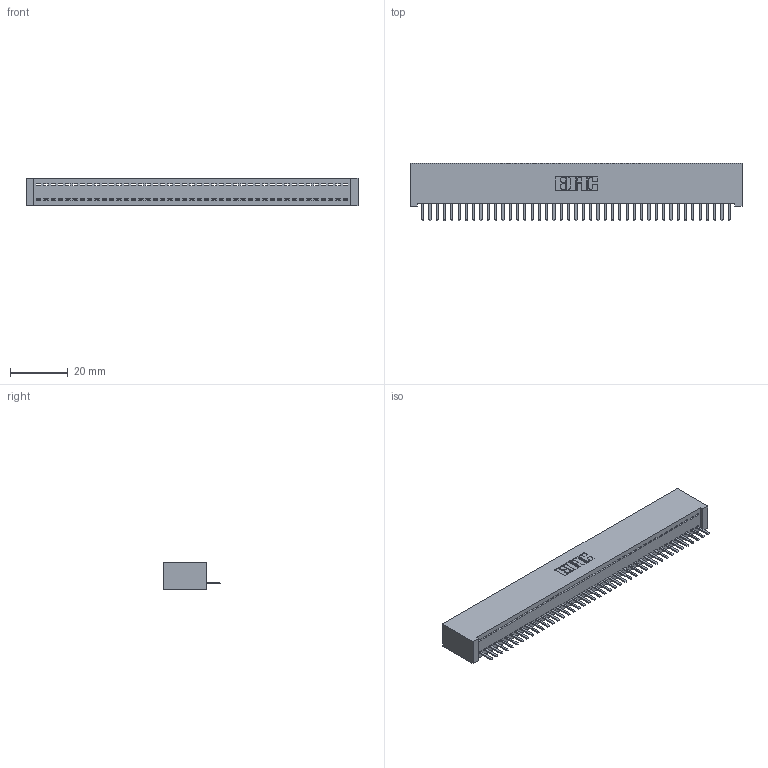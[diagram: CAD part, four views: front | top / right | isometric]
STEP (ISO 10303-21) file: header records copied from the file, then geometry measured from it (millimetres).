
FILE_DESCRIPTION (( 'STEP AP203' ), '1' );
FILE_NAME ('392-043-520-101.STEP', '2018-08-16T14:11:00', ( '' ), ( '' ), 'SwSTEP 2.0', 'SolidWorks 2016', '' );
FILE_SCHEMA (( 'CONFIG_CONTROL_DESIGN' ));
Length unit declared in the file: inch
Products named in the file (3): 342 Part_Lugless; 345-292-001_345-293-120; 392-043-520-101
Assembly tree (44 placements, depth 2):
  392-043-520-101
    342 Part_Lugless
    345-292-001_345-293-120  x43
Bounding box: 115.47 x 20.02 x 9.4 mm (x, y, z)
Volume: 10413.2 mm3; surface area: 15237.7 mm2
Topology: 44 solids, 44 shells, 2768 faces, 8187 edges, 5342 vertices
Faces by surface type: plane 1954, cylinder 814
Entity records: 25863 total; most frequent: CARTESIAN_POINT 4479, ORIENTED_EDGE 4446, DIRECTION 3757, EDGE_CURVE 2223, LINE 2099, VECTOR 2099, VERTEX_POINT 1478, AXIS2_PLACEMENT_3D 829
